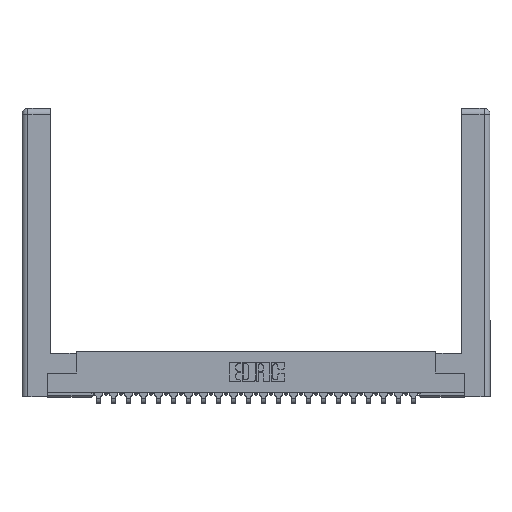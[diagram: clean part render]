
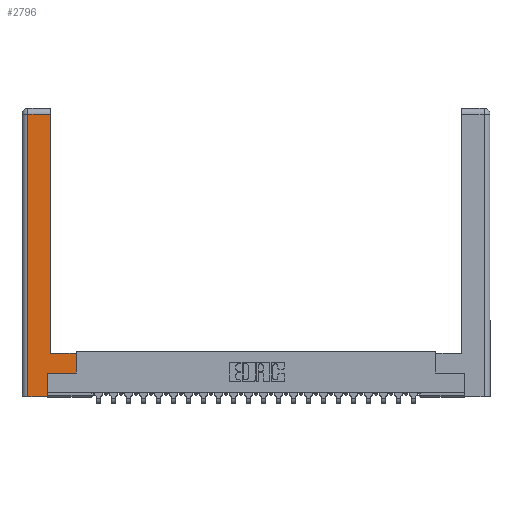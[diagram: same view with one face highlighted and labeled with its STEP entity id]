
A CAD part, top view. The second image highlights one B-rep face of the part: STEP entity #2796.
In plain terms, the highlighted planar face has unit normal (0, 0, 1).
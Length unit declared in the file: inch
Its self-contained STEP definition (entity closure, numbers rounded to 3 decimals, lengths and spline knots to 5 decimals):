
#115 = VERTEX_POINT ( 'NONE', #19729 ) ;
#629 = AXIS2_PLACEMENT_3D ( 'NONE', #8716, #21748, #5067 ) ;
#856 = EDGE_CURVE ( 'NONE', #1406, #115, #22613, .T. ) ;
#1157 = EDGE_CURVE ( 'NONE', #115, #15417, #7613, .T. ) ;
#1406 = VERTEX_POINT ( 'NONE', #14187 ) ;
#1669 = ORIENTED_EDGE ( 'NONE', *, *, #19206, .T. ) ;
#1973 = VECTOR ( 'NONE', #6660, 39.37008 ) ;
#2009 = CARTESIAN_POINT ( 'NONE',  ( 0.565, 0.245, 0. ) ) ;
#2113 = EDGE_LOOP ( 'NONE', ( #18920, #17952, #4960, #4594, #1669, #15200, #22347, #6380 ) ) ;
#2197 = CARTESIAN_POINT ( 'NONE',  ( 0.565, 0.45, 0. ) ) ;
#2796 = ADVANCED_FACE ( 'NONE', ( #3131 ), #17959, .F. ) ;
#2893 = EDGE_CURVE ( 'NONE', #11869, #4268, #7248, .T. ) ;
#3131 = FACE_OUTER_BOUND ( 'NONE', #2113, .T. ) ;
#3707 = DIRECTION ( 'NONE',  ( 1., 0., 0. ) ) ;
#3867 = CARTESIAN_POINT ( 'NONE',  ( 0.295, 0.45, 0. ) ) ;
#4074 = EDGE_CURVE ( 'NONE', #17543, #16709, #5071, .T. ) ;
#4268 = VERTEX_POINT ( 'NONE', #16494 ) ;
#4594 = ORIENTED_EDGE ( 'NONE', *, *, #20479, .T. ) ;
#4948 = EDGE_CURVE ( 'NONE', #4268, #17543, #23530, .T. ) ;
#4960 = ORIENTED_EDGE ( 'NONE', *, *, #1157, .T. ) ;
#5067 = DIRECTION ( 'NONE',  ( -1., 0., 0. ) ) ;
#5071 = LINE ( 'NONE', #21981, #1973 ) ;
#5185 = VECTOR ( 'NONE', #3707, 39.37008 ) ;
#5318 = DIRECTION ( 'NONE',  ( 0., -1., 0. ) ) ;
#6177 = CARTESIAN_POINT ( 'NONE',  ( 0.0615, 2.94, 0. ) ) ;
#6289 = VECTOR ( 'NONE', #7425, 39.37008 ) ;
#6325 = VECTOR ( 'NONE', #19395, 39.37008 ) ;
#6380 = ORIENTED_EDGE ( 'NONE', *, *, #4074, .T. ) ;
#6660 = DIRECTION ( 'NONE',  ( -1., 0., 0. ) ) ;
#7248 = LINE ( 'NONE', #2009, #5185 ) ;
#7425 = DIRECTION ( 'NONE',  ( 1., 0., 0. ) ) ;
#7613 = LINE ( 'NONE', #11026, #16033 ) ;
#8119 = CARTESIAN_POINT ( 'NONE',  ( 0.265, 0.245, 0. ) ) ;
#8202 = VECTOR ( 'NONE', #17495, 39.37008 ) ;
#8716 = CARTESIAN_POINT ( 'NONE',  ( 0., 0., 0. ) ) ;
#9104 = DIRECTION ( 'NONE',  ( 0., 1., 0. ) ) ;
#9898 = VECTOR ( 'NONE', #15084, 39.37008 ) ;
#10915 = VECTOR ( 'NONE', #9104, 39.37008 ) ;
#11026 = CARTESIAN_POINT ( 'NONE',  ( 0.0615, 0., 0. ) ) ;
#11296 = CARTESIAN_POINT ( 'NONE',  ( 0.565, 0.45, 0. ) ) ;
#11843 = CARTESIAN_POINT ( 'NONE',  ( 0.295, 3., 0. ) ) ;
#11869 = VERTEX_POINT ( 'NONE', #8119 ) ;
#12908 = CARTESIAN_POINT ( 'NONE',  ( 0.265, 0., 0. ) ) ;
#14187 = CARTESIAN_POINT ( 'NONE',  ( 0.295, 2.94, 0. ) ) ;
#14572 = CARTESIAN_POINT ( 'NONE',  ( 0.0615, 0., 0. ) ) ;
#14710 = CARTESIAN_POINT ( 'NONE',  ( 0.265, 0., 0. ) ) ;
#14921 = LINE ( 'NONE', #24084, #10915 ) ;
#15084 = DIRECTION ( 'NONE',  ( 0., 1., 0. ) ) ;
#15200 = ORIENTED_EDGE ( 'NONE', *, *, #2893, .T. ) ;
#15417 = VERTEX_POINT ( 'NONE', #14572 ) ;
#16033 = VECTOR ( 'NONE', #5318, 39.37008 ) ;
#16494 = CARTESIAN_POINT ( 'NONE',  ( 0.565, 0.245, 0. ) ) ;
#16709 = VERTEX_POINT ( 'NONE', #3867 ) ;
#17495 = DIRECTION ( 'NONE',  ( -1., 0., 0. ) ) ;
#17543 = VERTEX_POINT ( 'NONE', #11296 ) ;
#17952 = ORIENTED_EDGE ( 'NONE', *, *, #856, .T. ) ;
#17959 = PLANE ( 'NONE',  #629 ) ;
#18434 = LINE ( 'NONE', #11843, #6325 ) ;
#18920 = ORIENTED_EDGE ( 'NONE', *, *, #20959, .T. ) ;
#19206 = EDGE_CURVE ( 'NONE', #22205, #11869, #14921, .T. ) ;
#19395 = DIRECTION ( 'NONE',  ( 0., 1., 0. ) ) ;
#19729 = CARTESIAN_POINT ( 'NONE',  ( 0.0615, 2.94, 0. ) ) ;
#20098 = LINE ( 'NONE', #12908, #6289 ) ;
#20479 = EDGE_CURVE ( 'NONE', #15417, #22205, #20098, .T. ) ;
#20959 = EDGE_CURVE ( 'NONE', #16709, #1406, #18434, .T. ) ;
#21748 = DIRECTION ( 'NONE',  ( 0., 0., -1. ) ) ;
#21981 = CARTESIAN_POINT ( 'NONE',  ( 0.295, 0.45, 0. ) ) ;
#22205 = VERTEX_POINT ( 'NONE', #14710 ) ;
#22347 = ORIENTED_EDGE ( 'NONE', *, *, #4948, .T. ) ;
#22613 = LINE ( 'NONE', #6177, #8202 ) ;
#23530 = LINE ( 'NONE', #2197, #9898 ) ;
#24084 = CARTESIAN_POINT ( 'NONE',  ( 0.265, 0.245, 0. ) ) ;
